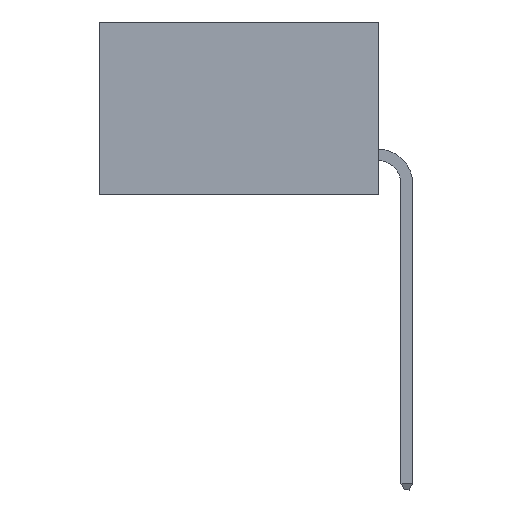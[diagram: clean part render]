
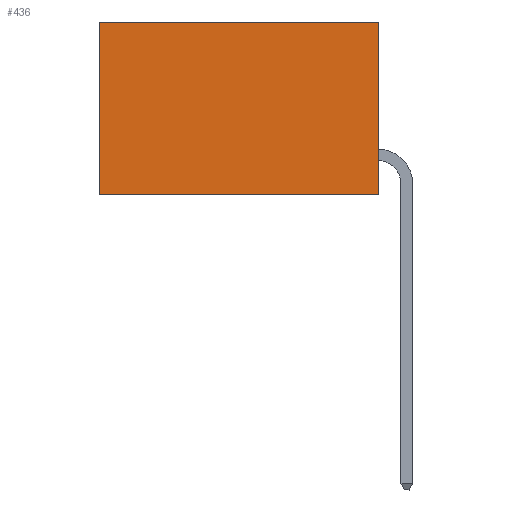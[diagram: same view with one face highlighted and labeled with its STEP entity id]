
A CAD part, left-side view. The second image highlights one B-rep face of the part: STEP entity #436.
In plain terms, the highlighted planar face has unit normal (-1, 0, 0).
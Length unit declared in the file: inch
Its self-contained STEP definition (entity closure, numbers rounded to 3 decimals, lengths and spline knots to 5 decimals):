
#436 = ADVANCED_FACE ( 'NONE', ( #17845 ), #17861, .F. ) ;
#805 = ORIENTED_EDGE ( 'NONE', *, *, #18694, .F. ) ;
#1621 = ORIENTED_EDGE ( 'NONE', *, *, #9806, .T. ) ;
#1845 = DIRECTION ( 'NONE',  ( 0., 0., -1. ) ) ;
#1886 = CARTESIAN_POINT ( 'NONE',  ( 0.298, 0., -0.37 ) ) ;
#2255 = VERTEX_POINT ( 'NONE', #1886 ) ;
#3857 = EDGE_LOOP ( 'NONE', ( #8184, #7940, #805, #1621 ) ) ;
#3959 = DIRECTION ( 'NONE',  ( 0., 1., 0. ) ) ;
#3986 = VECTOR ( 'NONE', #9685, 39.37008 ) ;
#4743 = CARTESIAN_POINT ( 'NONE',  ( 0.298, 0.6, 0. ) ) ;
#5502 = VECTOR ( 'NONE', #9548, 39.37008 ) ;
#6433 = LINE ( 'NONE', #6573, #5502 ) ;
#6573 = CARTESIAN_POINT ( 'NONE',  ( 0.298, 0., -0.37 ) ) ;
#6664 = VERTEX_POINT ( 'NONE', #16477 ) ;
#7273 = VECTOR ( 'NONE', #1845, 39.37008 ) ;
#7548 = CARTESIAN_POINT ( 'NONE',  ( 0.298, 0., 0. ) ) ;
#7940 = ORIENTED_EDGE ( 'NONE', *, *, #16669, .F. ) ;
#7985 = LINE ( 'NONE', #15394, #3986 ) ;
#8153 = LINE ( 'NONE', #7548, #15348 ) ;
#8184 = ORIENTED_EDGE ( 'NONE', *, *, #14017, .T. ) ;
#9548 = DIRECTION ( 'NONE',  ( 0., 1., 0. ) ) ;
#9685 = DIRECTION ( 'NONE',  ( 0., 0., -1. ) ) ;
#9806 = EDGE_CURVE ( 'NONE', #6664, #12888, #8153, .T. ) ;
#10572 = VERTEX_POINT ( 'NONE', #16038 ) ;
#11951 = AXIS2_PLACEMENT_3D ( 'NONE', #14166, #17190, #12071 ) ;
#12071 = DIRECTION ( 'NONE',  ( 0., 0., -1. ) ) ;
#12888 = VERTEX_POINT ( 'NONE', #18394 ) ;
#14017 = EDGE_CURVE ( 'NONE', #12888, #10572, #18691, .T. ) ;
#14166 = CARTESIAN_POINT ( 'NONE',  ( 0.298, 0., 0. ) ) ;
#15348 = VECTOR ( 'NONE', #3959, 39.37008 ) ;
#15394 = CARTESIAN_POINT ( 'NONE',  ( 0.298, 0., 0. ) ) ;
#16038 = CARTESIAN_POINT ( 'NONE',  ( 0.298, 0.6, -0.37 ) ) ;
#16477 = CARTESIAN_POINT ( 'NONE',  ( 0.298, 0., 0. ) ) ;
#16669 = EDGE_CURVE ( 'NONE', #2255, #10572, #6433, .T. ) ;
#17190 = DIRECTION ( 'NONE',  ( 1., 0., 0. ) ) ;
#17845 = FACE_OUTER_BOUND ( 'NONE', #3857, .T. ) ;
#17861 = PLANE ( 'NONE',  #11951 ) ;
#18394 = CARTESIAN_POINT ( 'NONE',  ( 0.298, 0.6, 0. ) ) ;
#18691 = LINE ( 'NONE', #4743, #7273 ) ;
#18694 = EDGE_CURVE ( 'NONE', #6664, #2255, #7985, .T. ) ;
